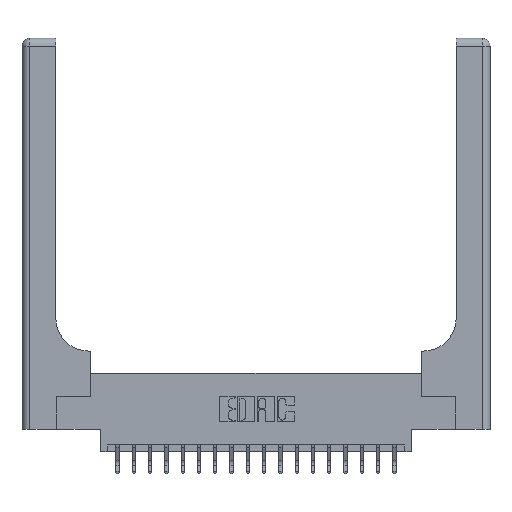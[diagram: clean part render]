
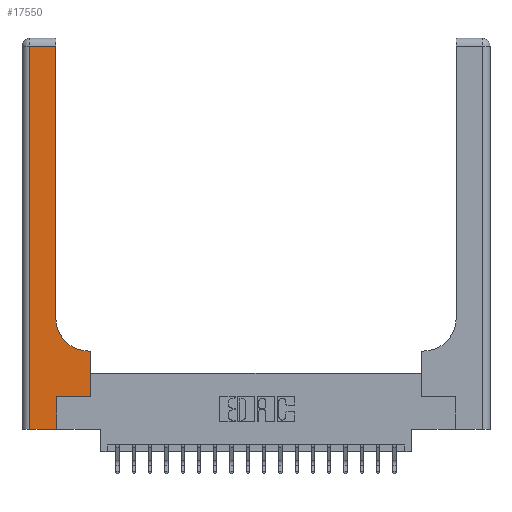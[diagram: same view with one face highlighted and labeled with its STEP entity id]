
A CAD part, top view. The second image highlights one B-rep face of the part: STEP entity #17550.
In plain terms, the highlighted planar face has unit normal (0, 0, 1).
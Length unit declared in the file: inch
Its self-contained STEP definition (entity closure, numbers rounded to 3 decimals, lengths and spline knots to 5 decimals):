
#53 = CARTESIAN_POINT ( 'NONE',  ( 0.528, 0.25, 0.37 ) ) ;
#502 = VECTOR ( 'NONE', #8185, 39.37008 ) ;
#682 = LINE ( 'NONE', #7939, #12919 ) ;
#686 = ORIENTED_EDGE ( 'NONE', *, *, #4644, .T. ) ;
#1673 = CARTESIAN_POINT ( 'NONE',  ( 0.06, 2.94, 0.37 ) ) ;
#2414 = CARTESIAN_POINT ( 'NONE',  ( 0.265, 0.25, 0.37 ) ) ;
#2734 = VECTOR ( 'NONE', #17910, 39.37008 ) ;
#2863 = VERTEX_POINT ( 'NONE', #9934 ) ;
#3049 = DIRECTION ( 'NONE',  ( 0., 0., -1. ) ) ;
#3092 = LINE ( 'NONE', #13960, #14771 ) ;
#3707 = VERTEX_POINT ( 'NONE', #19941 ) ;
#4001 = ORIENTED_EDGE ( 'NONE', *, *, #17818, .T. ) ;
#4072 = EDGE_CURVE ( 'NONE', #20447, #3707, #16134, .T. ) ;
#4470 = DIRECTION ( 'NONE',  ( 0., 1., 0. ) ) ;
#4644 = EDGE_CURVE ( 'NONE', #5753, #7930, #18307, .T. ) ;
#5709 = EDGE_CURVE ( 'NONE', #13645, #20152, #682, .T. ) ;
#5741 = VECTOR ( 'NONE', #11370, 39.37008 ) ;
#5753 = VERTEX_POINT ( 'NONE', #9615 ) ;
#5761 = CARTESIAN_POINT ( 'NONE',  ( 0.265, 0.25, 0.37 ) ) ;
#5847 = DIRECTION ( 'NONE',  ( 1., 0., 0. ) ) ;
#6495 = ORIENTED_EDGE ( 'NONE', *, *, #12565, .T. ) ;
#6837 = EDGE_LOOP ( 'NONE', ( #18777, #16106, #4001, #12922, #686, #13919, #6495, #15602, #19742 ) ) ;
#6948 = CARTESIAN_POINT ( 'NONE',  ( 0.51, 0.85, 0.37 ) ) ;
#6999 = LINE ( 'NONE', #13194, #2734 ) ;
#7587 = CARTESIAN_POINT ( 'NONE',  ( 0.528, 0.6, 0.37 ) ) ;
#7686 = VECTOR ( 'NONE', #16685, 39.37008 ) ;
#7721 = VERTEX_POINT ( 'NONE', #11676 ) ;
#7930 = VERTEX_POINT ( 'NONE', #5761 ) ;
#7939 = CARTESIAN_POINT ( 'NONE',  ( 0., 2.94, 0.37 ) ) ;
#8185 = DIRECTION ( 'NONE',  ( -1., 0., 0. ) ) ;
#8550 = DIRECTION ( 'NONE',  ( 1., 0., 0. ) ) ;
#9065 = LINE ( 'NONE', #16017, #502 ) ;
#9548 = DIRECTION ( 'NONE',  ( -1., 0., 0. ) ) ;
#9615 = CARTESIAN_POINT ( 'NONE',  ( 0.265, 0., 0.37 ) ) ;
#9795 = CARTESIAN_POINT ( 'NONE',  ( 0.265, 0., 0.37 ) ) ;
#9934 = CARTESIAN_POINT ( 'NONE',  ( 0.528, 0.25, 0.37 ) ) ;
#10874 = EDGE_CURVE ( 'NONE', #3707, #13645, #3092, .T. ) ;
#10971 = CARTESIAN_POINT ( 'NONE',  ( 0.26, 2.94, 0.37 ) ) ;
#11370 = DIRECTION ( 'NONE',  ( 0., 1., 0. ) ) ;
#11478 = FACE_OUTER_BOUND ( 'NONE', #6837, .T. ) ;
#11676 = CARTESIAN_POINT ( 'NONE',  ( 0.06, 0., 0.37 ) ) ;
#11952 = CARTESIAN_POINT ( 'NONE',  ( 0.51, 0.6, 0.37 ) ) ;
#12168 = CARTESIAN_POINT ( 'NONE',  ( 0., 0., 0.37 ) ) ;
#12380 = LINE ( 'NONE', #2414, #7686 ) ;
#12565 = EDGE_CURVE ( 'NONE', #2863, #12992, #18110, .T. ) ;
#12578 = CARTESIAN_POINT ( 'NONE',  ( 0., 3., 0.37 ) ) ;
#12919 = VECTOR ( 'NONE', #9548, 39.37008 ) ;
#12922 = ORIENTED_EDGE ( 'NONE', *, *, #17934, .T. ) ;
#12992 = VERTEX_POINT ( 'NONE', #7587 ) ;
#13194 = CARTESIAN_POINT ( 'NONE',  ( 0.06, 3., 0.37 ) ) ;
#13645 = VERTEX_POINT ( 'NONE', #10971 ) ;
#13743 = AXIS2_PLACEMENT_3D ( 'NONE', #6948, #17948, #8550 ) ;
#13919 = ORIENTED_EDGE ( 'NONE', *, *, #19756, .T. ) ;
#13960 = CARTESIAN_POINT ( 'NONE',  ( 0.26, 3., 0.37 ) ) ;
#14169 = DIRECTION ( 'NONE',  ( -1., 0., 0. ) ) ;
#14364 = DIRECTION ( 'NONE',  ( 0., 1., 0. ) ) ;
#14454 = VECTOR ( 'NONE', #14364, 39.37008 ) ;
#14771 = VECTOR ( 'NONE', #4470, 39.37008 ) ;
#15602 = ORIENTED_EDGE ( 'NONE', *, *, #16225, .T. ) ;
#16017 = CARTESIAN_POINT ( 'NONE',  ( 0.26, 0.6, 0.37 ) ) ;
#16106 = ORIENTED_EDGE ( 'NONE', *, *, #5709, .T. ) ;
#16134 = CIRCLE ( 'NONE', #13743, 0.25 ) ;
#16225 = EDGE_CURVE ( 'NONE', #12992, #20447, #9065, .T. ) ;
#16645 = AXIS2_PLACEMENT_3D ( 'NONE', #12578, #3049, #14169 ) ;
#16685 = DIRECTION ( 'NONE',  ( 1., 0., 0. ) ) ;
#17550 = ADVANCED_FACE ( 'NONE', ( #11478 ), #20303, .F. ) ;
#17580 = VECTOR ( 'NONE', #5847, 39.37008 ) ;
#17818 = EDGE_CURVE ( 'NONE', #20152, #7721, #6999, .T. ) ;
#17910 = DIRECTION ( 'NONE',  ( 0., -1., 0. ) ) ;
#17934 = EDGE_CURVE ( 'NONE', #7721, #5753, #19037, .T. ) ;
#17948 = DIRECTION ( 'NONE',  ( 0., 0., -1. ) ) ;
#18110 = LINE ( 'NONE', #53, #14454 ) ;
#18307 = LINE ( 'NONE', #9795, #5741 ) ;
#18777 = ORIENTED_EDGE ( 'NONE', *, *, #10874, .T. ) ;
#19037 = LINE ( 'NONE', #12168, #17580 ) ;
#19742 = ORIENTED_EDGE ( 'NONE', *, *, #4072, .T. ) ;
#19756 = EDGE_CURVE ( 'NONE', #7930, #2863, #12380, .T. ) ;
#19941 = CARTESIAN_POINT ( 'NONE',  ( 0.26, 0.85, 0.37 ) ) ;
#20152 = VERTEX_POINT ( 'NONE', #1673 ) ;
#20303 = PLANE ( 'NONE',  #16645 ) ;
#20447 = VERTEX_POINT ( 'NONE', #11952 ) ;
